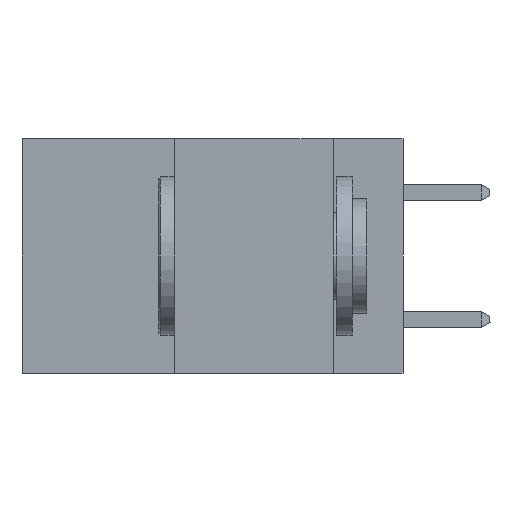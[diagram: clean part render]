
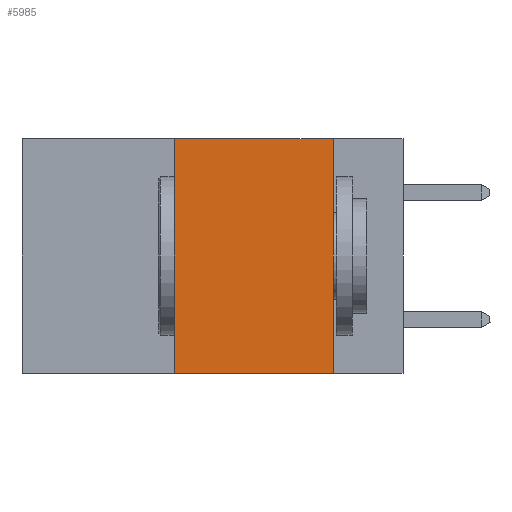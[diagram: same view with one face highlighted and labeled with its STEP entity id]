
A CAD part, left-side view. The second image highlights one B-rep face of the part: STEP entity #5985.
In plain terms, the highlighted planar face has unit normal (-1, 0, 0).
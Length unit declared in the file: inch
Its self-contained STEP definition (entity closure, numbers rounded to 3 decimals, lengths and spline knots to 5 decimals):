
#1197 = DIRECTION ( 'NONE',  ( 0., 0., -1. ) ) ;
#1537 = VECTOR ( 'NONE', #1197, 39.37008 ) ;
#1732 = ORIENTED_EDGE ( 'NONE', *, *, #2682, .T. ) ;
#2027 = CARTESIAN_POINT ( 'NONE',  ( 0., 0.36, 0. ) ) ;
#2196 = LINE ( 'NONE', #8514, #1537 ) ;
#2682 = EDGE_CURVE ( 'NONE', #13361, #7981, #3461, .T. ) ;
#3054 = DIRECTION ( 'NONE',  ( 0., 0., 1. ) ) ;
#3461 = LINE ( 'NONE', #12712, #8563 ) ;
#3510 = VERTEX_POINT ( 'NONE', #5119 ) ;
#3878 = CARTESIAN_POINT ( 'NONE',  ( 0., 0.36, -0.37 ) ) ;
#4290 = EDGE_CURVE ( 'NONE', #8616, #3510, #6293, .T. ) ;
#4382 = VECTOR ( 'NONE', #3054, 39.37008 ) ;
#5119 = CARTESIAN_POINT ( 'NONE',  ( 0., 0.11, 0. ) ) ;
#5430 = DIRECTION ( 'NONE',  ( 0., 0., -1. ) ) ;
#5592 = DIRECTION ( 'NONE',  ( 1., 0., 0. ) ) ;
#5637 = CARTESIAN_POINT ( 'NONE',  ( 0., 0.6, 0. ) ) ;
#5888 = PLANE ( 'NONE',  #13321 ) ;
#5985 = ADVANCED_FACE ( 'NONE', ( #12898 ), #5888, .F. ) ;
#6205 = CARTESIAN_POINT ( 'NONE',  ( 0., 0.11, -0.37 ) ) ;
#6293 = LINE ( 'NONE', #8969, #11768 ) ;
#6417 = ORIENTED_EDGE ( 'NONE', *, *, #10095, .F. ) ;
#7130 = LINE ( 'NONE', #13385, #4382 ) ;
#7491 = ORIENTED_EDGE ( 'NONE', *, *, #4290, .F. ) ;
#7981 = VERTEX_POINT ( 'NONE', #6205 ) ;
#8514 = CARTESIAN_POINT ( 'NONE',  ( 0., 0.11, 0. ) ) ;
#8563 = VECTOR ( 'NONE', #12348, 39.37008 ) ;
#8616 = VERTEX_POINT ( 'NONE', #2027 ) ;
#8969 = CARTESIAN_POINT ( 'NONE',  ( 0., 0.6, 0. ) ) ;
#9082 = DIRECTION ( 'NONE',  ( 0., -1., 0. ) ) ;
#10095 = EDGE_CURVE ( 'NONE', #3510, #7981, #2196, .T. ) ;
#10541 = EDGE_CURVE ( 'NONE', #13361, #8616, #7130, .T. ) ;
#10837 = ORIENTED_EDGE ( 'NONE', *, *, #10541, .F. ) ;
#11768 = VECTOR ( 'NONE', #9082, 39.37008 ) ;
#12348 = DIRECTION ( 'NONE',  ( 0., -1., 0. ) ) ;
#12385 = EDGE_LOOP ( 'NONE', ( #6417, #7491, #10837, #1732 ) ) ;
#12712 = CARTESIAN_POINT ( 'NONE',  ( 0., 0.6, -0.37 ) ) ;
#12898 = FACE_OUTER_BOUND ( 'NONE', #12385, .T. ) ;
#13321 = AXIS2_PLACEMENT_3D ( 'NONE', #5637, #5592, #5430 ) ;
#13361 = VERTEX_POINT ( 'NONE', #3878 ) ;
#13385 = CARTESIAN_POINT ( 'NONE',  ( 0., 0.36, 0. ) ) ;
